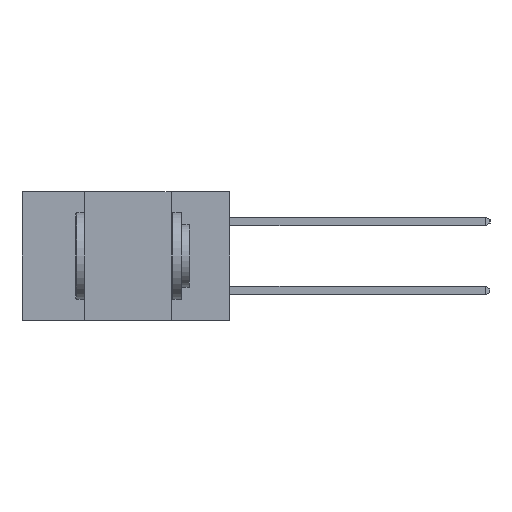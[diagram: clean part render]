
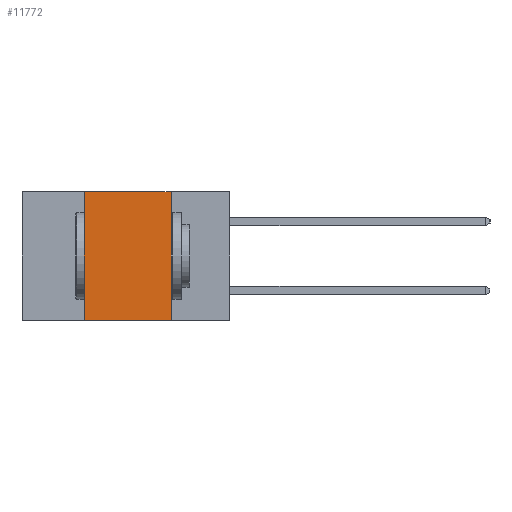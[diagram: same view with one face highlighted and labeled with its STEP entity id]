
A CAD part, left-side view. The second image highlights one B-rep face of the part: STEP entity #11772.
In plain terms, the highlighted planar face has unit normal (-1, 0, 0).
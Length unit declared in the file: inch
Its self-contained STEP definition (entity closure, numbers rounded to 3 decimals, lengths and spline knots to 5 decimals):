
#478 = VECTOR ( 'NONE', #12979, 39.37008 ) ;
#536 = EDGE_CURVE ( 'NONE', #8758, #5095, #11801, .T. ) ;
#1227 = DIRECTION ( 'NONE',  ( 0., -1., 0. ) ) ;
#1538 = ORIENTED_EDGE ( 'NONE', *, *, #6480, .F. ) ;
#1550 = DIRECTION ( 'NONE',  ( 0., 0., 1. ) ) ;
#1566 = CARTESIAN_POINT ( 'NONE',  ( 0., 0.42, 0. ) ) ;
#1897 = ORIENTED_EDGE ( 'NONE', *, *, #2076, .T. ) ;
#2076 = EDGE_CURVE ( 'NONE', #8758, #3279, #13920, .T. ) ;
#2529 = VECTOR ( 'NONE', #1550, 39.37008 ) ;
#2977 = CARTESIAN_POINT ( 'NONE',  ( 0., 0.6, 0. ) ) ;
#3279 = VERTEX_POINT ( 'NONE', #4578 ) ;
#3363 = LINE ( 'NONE', #3699, #9100 ) ;
#3699 = CARTESIAN_POINT ( 'NONE',  ( 0., 0.17, 0. ) ) ;
#4475 = DIRECTION ( 'NONE',  ( 0., 0., -1. ) ) ;
#4578 = CARTESIAN_POINT ( 'NONE',  ( 0., 0.17, -0.37 ) ) ;
#4579 = ORIENTED_EDGE ( 'NONE', *, *, #7147, .F. ) ;
#5095 = VERTEX_POINT ( 'NONE', #6866 ) ;
#5175 = VECTOR ( 'NONE', #1227, 39.37008 ) ;
#5296 = PLANE ( 'NONE',  #7605 ) ;
#6443 = DIRECTION ( 'NONE',  ( 1., 0., 0. ) ) ;
#6480 = EDGE_CURVE ( 'NONE', #11930, #3279, #3363, .T. ) ;
#6866 = CARTESIAN_POINT ( 'NONE',  ( 0., 0.42, 0. ) ) ;
#7147 = EDGE_CURVE ( 'NONE', #5095, #11930, #9590, .T. ) ;
#7605 = AXIS2_PLACEMENT_3D ( 'NONE', #2977, #6443, #14065 ) ;
#8088 = CARTESIAN_POINT ( 'NONE',  ( 0., 0.42, -0.37 ) ) ;
#8396 = FACE_OUTER_BOUND ( 'NONE', #9794, .T. ) ;
#8758 = VERTEX_POINT ( 'NONE', #8088 ) ;
#8829 = CARTESIAN_POINT ( 'NONE',  ( 0., 0.6, -0.37 ) ) ;
#8988 = CARTESIAN_POINT ( 'NONE',  ( 0., 0.17, 0. ) ) ;
#9100 = VECTOR ( 'NONE', #4475, 39.37008 ) ;
#9590 = LINE ( 'NONE', #13223, #478 ) ;
#9794 = EDGE_LOOP ( 'NONE', ( #1538, #4579, #10569, #1897 ) ) ;
#10569 = ORIENTED_EDGE ( 'NONE', *, *, #536, .F. ) ;
#11772 = ADVANCED_FACE ( 'NONE', ( #8396 ), #5296, .F. ) ;
#11801 = LINE ( 'NONE', #1566, #2529 ) ;
#11930 = VERTEX_POINT ( 'NONE', #8988 ) ;
#12979 = DIRECTION ( 'NONE',  ( 0., -1., 0. ) ) ;
#13223 = CARTESIAN_POINT ( 'NONE',  ( 0., 0.6, 0. ) ) ;
#13920 = LINE ( 'NONE', #8829, #5175 ) ;
#14065 = DIRECTION ( 'NONE',  ( 0., 0., -1. ) ) ;
